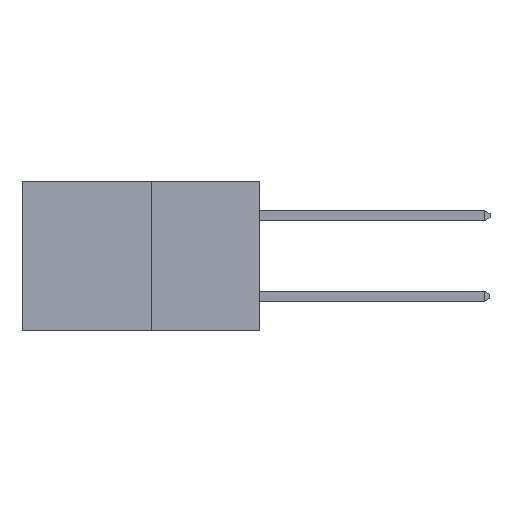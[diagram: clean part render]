
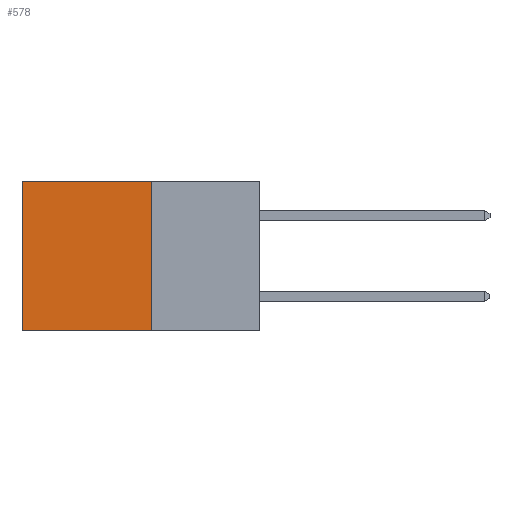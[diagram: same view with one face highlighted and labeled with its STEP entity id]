
A CAD part, left-side view. The second image highlights one B-rep face of the part: STEP entity #578.
In plain terms, the highlighted planar face has unit normal (-1, 0, 0).
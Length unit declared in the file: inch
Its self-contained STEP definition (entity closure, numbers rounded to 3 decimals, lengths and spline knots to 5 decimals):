
#578 = ADVANCED_FACE ( 'NONE', ( #1229 ), #7419, .F. ) ;
#803 = ORIENTED_EDGE ( 'NONE', *, *, #6903, .F. ) ;
#1229 = FACE_OUTER_BOUND ( 'NONE', #2830, .T. ) ;
#1419 = CARTESIAN_POINT ( 'NONE',  ( 0.277, 0.27, -0.37 ) ) ;
#1487 = DIRECTION ( 'NONE',  ( 1., 0., 0. ) ) ;
#1494 = VERTEX_POINT ( 'NONE', #5413 ) ;
#1653 = EDGE_CURVE ( 'NONE', #3210, #3298, #6678, .T. ) ;
#1727 = DIRECTION ( 'NONE',  ( 0., 0., -1. ) ) ;
#2201 = DIRECTION ( 'NONE',  ( 0., 1., 0. ) ) ;
#2250 = DIRECTION ( 'NONE',  ( 0., 0., -1. ) ) ;
#2536 = CARTESIAN_POINT ( 'NONE',  ( 0.277, 0.27, -0.37 ) ) ;
#2654 = LINE ( 'NONE', #3978, #4315 ) ;
#2661 = EDGE_CURVE ( 'NONE', #3298, #1494, #2654, .T. ) ;
#2701 = CARTESIAN_POINT ( 'NONE',  ( 0.277, 0.27, -0.37 ) ) ;
#2830 = EDGE_LOOP ( 'NONE', ( #3420, #3336, #803, #6005 ) ) ;
#2911 = CARTESIAN_POINT ( 'NONE',  ( 0.277, 0.59, 0. ) ) ;
#3210 = VERTEX_POINT ( 'NONE', #4237 ) ;
#3238 = VECTOR ( 'NONE', #8470, 39.37008 ) ;
#3269 = DIRECTION ( 'NONE',  ( 0., 0., -1. ) ) ;
#3298 = VERTEX_POINT ( 'NONE', #2911 ) ;
#3336 = ORIENTED_EDGE ( 'NONE', *, *, #8466, .F. ) ;
#3420 = ORIENTED_EDGE ( 'NONE', *, *, #2661, .T. ) ;
#3978 = CARTESIAN_POINT ( 'NONE',  ( 0.277, 0.59, -0.37 ) ) ;
#4237 = CARTESIAN_POINT ( 'NONE',  ( 0.277, 0.27, 0. ) ) ;
#4315 = VECTOR ( 'NONE', #2250, 39.37008 ) ;
#4458 = VERTEX_POINT ( 'NONE', #2701 ) ;
#4553 = LINE ( 'NONE', #2536, #7736 ) ;
#5138 = CARTESIAN_POINT ( 'NONE',  ( 0.277, 0.27, 0. ) ) ;
#5413 = CARTESIAN_POINT ( 'NONE',  ( 0.277, 0.59, -0.37 ) ) ;
#5773 = AXIS2_PLACEMENT_3D ( 'NONE', #6455, #1487, #1727 ) ;
#6005 = ORIENTED_EDGE ( 'NONE', *, *, #1653, .T. ) ;
#6455 = CARTESIAN_POINT ( 'NONE',  ( 0.277, 0.27, -0.37 ) ) ;
#6678 = LINE ( 'NONE', #5138, #3238 ) ;
#6903 = EDGE_CURVE ( 'NONE', #3210, #4458, #4553, .T. ) ;
#7403 = LINE ( 'NONE', #1419, #8738 ) ;
#7419 = PLANE ( 'NONE',  #5773 ) ;
#7736 = VECTOR ( 'NONE', #3269, 39.37008 ) ;
#8466 = EDGE_CURVE ( 'NONE', #4458, #1494, #7403, .T. ) ;
#8470 = DIRECTION ( 'NONE',  ( 0., 1., 0. ) ) ;
#8738 = VECTOR ( 'NONE', #2201, 39.37008 ) ;
